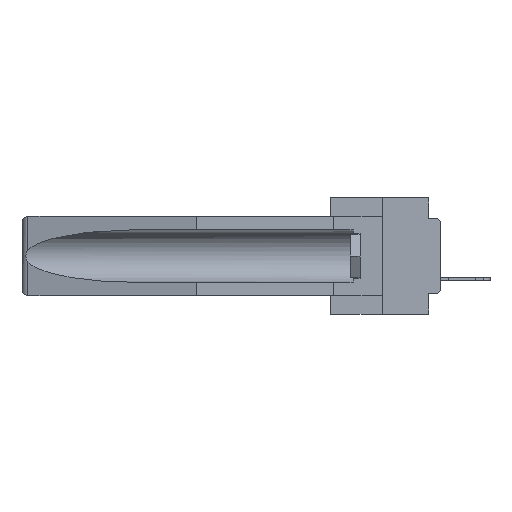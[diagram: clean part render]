
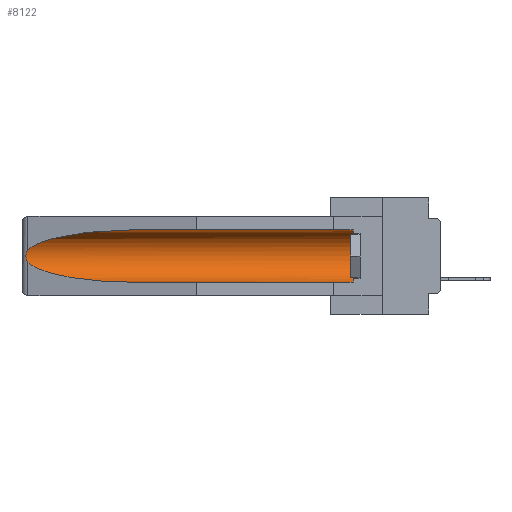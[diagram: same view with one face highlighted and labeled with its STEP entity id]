
A CAD part, left-side view. The second image highlights one B-rep face of the part: STEP entity #8122.
In plain terms, the highlighted cylindrical face has radius 2.857 mm (diameter 5.715 mm), a partial arc.
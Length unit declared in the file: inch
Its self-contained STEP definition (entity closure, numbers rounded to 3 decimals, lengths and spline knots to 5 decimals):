
#556 = CARTESIAN_POINT ( 'NONE',  ( 0.26597, 1.5296, -0.19026 ) ) ;
#621 = CARTESIAN_POINT ( 'NONE',  ( 0.155, -0.30754, -0.059 ) ) ;
#867 = CARTESIAN_POINT ( 'NONE',  ( 0.2675, 1.53308, -0.17534 ) ) ;
#1340 = LINE ( 'NONE', #23903, #28099 ) ;
#1613 = EDGE_CURVE ( 'NONE', #14143, #15477, #23474, .T. ) ;
#1787 = DIRECTION ( 'NONE',  ( 0., 1., 0. ) ) ;
#1848 = CARTESIAN_POINT ( 'NONE',  ( 0.26537, 1.52718, -0.19328 ) ) ;
#3108 = EDGE_CURVE ( 'NONE', #6608, #26891, #12330, .T. ) ;
#3466 = EDGE_LOOP ( 'NONE', ( #13901, #18626, #21581, #26061, #16546, #19455 ) ) ;
#3960 = CARTESIAN_POINT ( 'NONE',  ( 0.26597, 1.52961, -0.15275 ) ) ;
#5220 = EDGE_CURVE ( 'NONE', #14143, #26891, #1340, .T. ) ;
#5384 = CARTESIAN_POINT ( 'NONE',  ( 0.155, 1.07973, -0.059 ) ) ;
#6537 = VERTEX_POINT ( 'NONE', #7357 ) ;
#6608 = VERTEX_POINT ( 'NONE', #19957 ) ;
#6644 = AXIS2_PLACEMENT_3D ( 'NONE', #27509, #10367, #13088 ) ;
#6911 = CARTESIAN_POINT ( 'NONE',  ( 0.2673, 1.5327, -0.16383 ) ) ;
#7357 = CARTESIAN_POINT ( 'NONE',  ( 0.26537, 1.52718, -0.14972 ) ) ;
#8122 = ADVANCED_FACE ( 'NONE', ( #14846 ), #8445, .F. ) ;
#8445 = CYLINDRICAL_SURFACE ( 'NONE', #6644, 0.1125 ) ;
#8997 = CARTESIAN_POINT ( 'NONE',  ( 0.21114, 1.30732, -0.284 ) ) ;
#9334 = EDGE_CURVE ( 'NONE', #20909, #6537, #14636, .T. ) ;
#9435 = EDGE_CURVE ( 'NONE', #6537, #6608, #9999, .T. ) ;
#9999 = B_SPLINE_CURVE_WITH_KNOTS ( 'NONE', 3,
 ( #11150, #3960, #30675, #6911, #24697, #867, #17718, #24594, #556, #18350 ),
 .UNSPECIFIED., .F., .F.,
 ( 4, 2, 2, 2, 4 ),
 ( 0., 0.00029, 0.00058, 0.00087, 0.00117 ),
 .UNSPECIFIED. ) ;
#10367 = DIRECTION ( 'NONE',  ( 0., 1., 0. ) ) ;
#10689 = EDGE_CURVE ( 'NONE', #15477, #20909, #30862, .T. ) ;
#10738 = AXIS2_PLACEMENT_3D ( 'NONE', #29592, #20033, #22350 ) ;
#11150 = CARTESIAN_POINT ( 'NONE',  ( 0.26537, 1.52718, -0.14972 ) ) ;
#12330 =( BOUNDED_CURVE ( )  B_SPLINE_CURVE ( 3, ( #1848, #18593, #8997, #30560 ),
 .UNSPECIFIED., .F., .F. ) 
 B_SPLINE_CURVE_WITH_KNOTS ( ( 4, 4 ),
 ( 0.1948, 1.5708 ),
 .UNSPECIFIED. ) 
 CURVE ( )  GEOMETRIC_REPRESENTATION_ITEM ( )  RATIONAL_B_SPLINE_CURVE ( ( 1., 0.848, 0.848, 1. ) ) 
 REPRESENTATION_ITEM ( '' )  );
#13038 = CARTESIAN_POINT ( 'NONE',  ( 0.155, 0.126, -0.059 ) ) ;
#13088 = DIRECTION ( 'NONE',  ( 0., 0., 1. ) ) ;
#13901 = ORIENTED_EDGE ( 'NONE', *, *, #9334, .T. ) ;
#14143 = VERTEX_POINT ( 'NONE', #20230 ) ;
#14636 =( BOUNDED_CURVE ( )  B_SPLINE_CURVE ( 3, ( #5384, #15403, #29488, #15103 ),
 .UNSPECIFIED., .F., .F. ) 
 B_SPLINE_CURVE_WITH_KNOTS ( ( 4, 4 ),
 ( 4.71239, 6.08839 ),
 .UNSPECIFIED. ) 
 CURVE ( )  GEOMETRIC_REPRESENTATION_ITEM ( )  RATIONAL_B_SPLINE_CURVE ( ( 1., 0.848, 0.848, 1. ) ) 
 REPRESENTATION_ITEM ( '' )  );
#14675 = VECTOR ( 'NONE', #15456, 39.37008 ) ;
#14846 = FACE_OUTER_BOUND ( 'NONE', #3466, .T. ) ;
#15103 = CARTESIAN_POINT ( 'NONE',  ( 0.26537, 1.52718, -0.14972 ) ) ;
#15403 = CARTESIAN_POINT ( 'NONE',  ( 0.21114, 1.30732, -0.059 ) ) ;
#15456 = DIRECTION ( 'NONE',  ( 0., 1., 0. ) ) ;
#15477 = VERTEX_POINT ( 'NONE', #13038 ) ;
#16546 = ORIENTED_EDGE ( 'NONE', *, *, #1613, .T. ) ;
#17718 = CARTESIAN_POINT ( 'NONE',  ( 0.2673, 1.53269, -0.17917 ) ) ;
#18350 = CARTESIAN_POINT ( 'NONE',  ( 0.26537, 1.52718, -0.19328 ) ) ;
#18593 = CARTESIAN_POINT ( 'NONE',  ( 0.25451, 1.48313, -0.24835 ) ) ;
#18626 = ORIENTED_EDGE ( 'NONE', *, *, #9435, .T. ) ;
#19455 = ORIENTED_EDGE ( 'NONE', *, *, #10689, .T. ) ;
#19957 = CARTESIAN_POINT ( 'NONE',  ( 0.26537, 1.52718, -0.19328 ) ) ;
#20033 = DIRECTION ( 'NONE',  ( 0., -1., 0. ) ) ;
#20230 = CARTESIAN_POINT ( 'NONE',  ( 0.155, 0.126, -0.284 ) ) ;
#20909 = VERTEX_POINT ( 'NONE', #27482 ) ;
#21581 = ORIENTED_EDGE ( 'NONE', *, *, #3108, .T. ) ;
#22350 = DIRECTION ( 'NONE',  ( 0., 0., 1. ) ) ;
#23474 = CIRCLE ( 'NONE', #10738, 0.1125 ) ;
#23903 = CARTESIAN_POINT ( 'NONE',  ( 0.155, -0.30754, -0.284 ) ) ;
#24594 = CARTESIAN_POINT ( 'NONE',  ( 0.26655, 1.53094, -0.18657 ) ) ;
#24697 = CARTESIAN_POINT ( 'NONE',  ( 0.2675, 1.53308, -0.16763 ) ) ;
#26061 = ORIENTED_EDGE ( 'NONE', *, *, #5220, .F. ) ;
#26484 = CARTESIAN_POINT ( 'NONE',  ( 0.155, 1.07973, -0.284 ) ) ;
#26891 = VERTEX_POINT ( 'NONE', #26484 ) ;
#27482 = CARTESIAN_POINT ( 'NONE',  ( 0.155, 1.07973, -0.059 ) ) ;
#27509 = CARTESIAN_POINT ( 'NONE',  ( 0.155, -0.30754, -0.1715 ) ) ;
#28099 = VECTOR ( 'NONE', #1787, 39.37008 ) ;
#29488 = CARTESIAN_POINT ( 'NONE',  ( 0.25451, 1.48313, -0.09465 ) ) ;
#29592 = CARTESIAN_POINT ( 'NONE',  ( 0.155, 0.126, -0.1715 ) ) ;
#30560 = CARTESIAN_POINT ( 'NONE',  ( 0.155, 1.07973, -0.284 ) ) ;
#30675 = CARTESIAN_POINT ( 'NONE',  ( 0.26654, 1.53092, -0.15636 ) ) ;
#30862 = LINE ( 'NONE', #621, #14675 ) ;
